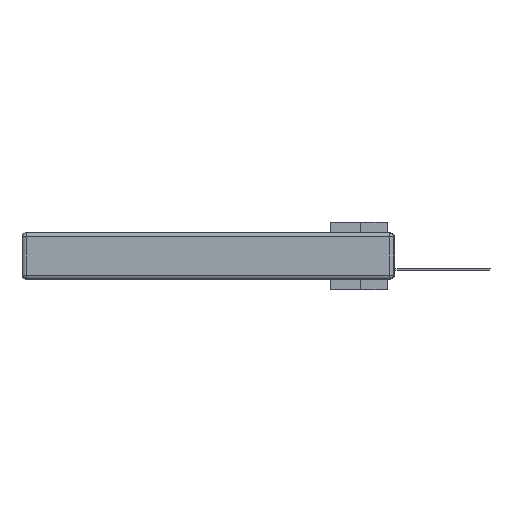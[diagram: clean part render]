
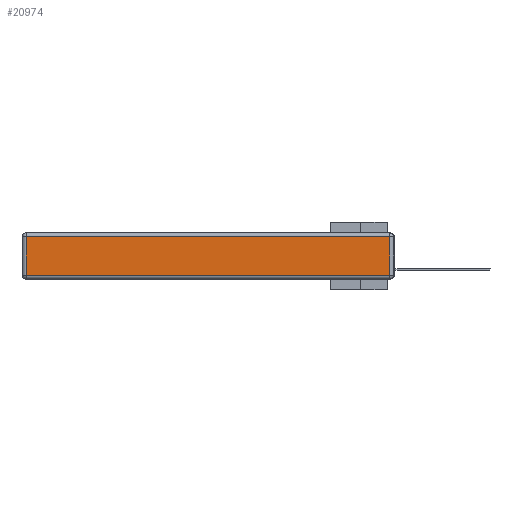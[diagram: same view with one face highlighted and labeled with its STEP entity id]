
A CAD part, left-side view. The second image highlights one B-rep face of the part: STEP entity #20974.
In plain terms, the highlighted planar face has unit normal (-1, 0, 0).
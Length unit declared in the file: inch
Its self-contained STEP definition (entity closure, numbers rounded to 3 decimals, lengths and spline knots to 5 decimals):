
#761 = VECTOR ( 'NONE', #27339, 39.37008 ) ;
#1589 = VECTOR ( 'NONE', #25922, 39.37008 ) ;
#2242 = PLANE ( 'NONE',  #30374 ) ;
#3369 = CARTESIAN_POINT ( 'NONE',  ( 0., 2.72, -0.313 ) ) ;
#3684 = EDGE_CURVE ( 'NONE', #26740, #18772, #24900, .T. ) ;
#3913 = DIRECTION ( 'NONE',  ( 0., -1., 0. ) ) ;
#5776 = EDGE_LOOP ( 'NONE', ( #15739, #10584, #27710, #9105 ) ) ;
#6708 = DIRECTION ( 'NONE',  ( 0., 1., 0. ) ) ;
#7446 = FACE_OUTER_BOUND ( 'NONE', #5776, .T. ) ;
#7836 = VECTOR ( 'NONE', #3913, 39.37008 ) ;
#9105 = ORIENTED_EDGE ( 'NONE', *, *, #3684, .T. ) ;
#9355 = VECTOR ( 'NONE', #6708, 39.37008 ) ;
#10584 = ORIENTED_EDGE ( 'NONE', *, *, #13278, .T. ) ;
#12025 = LINE ( 'NONE', #31526, #7836 ) ;
#13278 = EDGE_CURVE ( 'NONE', #18781, #29137, #26244, .T. ) ;
#13727 = CARTESIAN_POINT ( 'NONE',  ( 0., 0.03, -0.03 ) ) ;
#15739 = ORIENTED_EDGE ( 'NONE', *, *, #31503, .T. ) ;
#16780 = LINE ( 'NONE', #27013, #9355 ) ;
#16877 = DIRECTION ( 'NONE',  ( 0., 0., 1. ) ) ;
#17421 = CARTESIAN_POINT ( 'NONE',  ( 0., 2.72, -0.343 ) ) ;
#17637 = EDGE_CURVE ( 'NONE', #29137, #26740, #16780, .T. ) ;
#18762 = CARTESIAN_POINT ( 'NONE',  ( 0., 0.03, -0.343 ) ) ;
#18772 = VERTEX_POINT ( 'NONE', #3369 ) ;
#18781 = VERTEX_POINT ( 'NONE', #30198 ) ;
#20974 = ADVANCED_FACE ( 'NONE', ( #7446 ), #2242, .T. ) ;
#24526 = CARTESIAN_POINT ( 'NONE',  ( 0., 0., -0.343 ) ) ;
#24900 = LINE ( 'NONE', #17421, #761 ) ;
#25922 = DIRECTION ( 'NONE',  ( 0., 0., 1. ) ) ;
#26244 = LINE ( 'NONE', #18762, #1589 ) ;
#26740 = VERTEX_POINT ( 'NONE', #30286 ) ;
#27013 = CARTESIAN_POINT ( 'NONE',  ( 0., 2.75, -0.03 ) ) ;
#27281 = DIRECTION ( 'NONE',  ( -1., 0., 0. ) ) ;
#27339 = DIRECTION ( 'NONE',  ( 0., 0., -1. ) ) ;
#27710 = ORIENTED_EDGE ( 'NONE', *, *, #17637, .T. ) ;
#29137 = VERTEX_POINT ( 'NONE', #13727 ) ;
#30198 = CARTESIAN_POINT ( 'NONE',  ( 0., 0.03, -0.313 ) ) ;
#30286 = CARTESIAN_POINT ( 'NONE',  ( 0., 2.72, -0.03 ) ) ;
#30374 = AXIS2_PLACEMENT_3D ( 'NONE', #24526, #27281, #16877 ) ;
#31503 = EDGE_CURVE ( 'NONE', #18772, #18781, #12025, .T. ) ;
#31526 = CARTESIAN_POINT ( 'NONE',  ( 0., 0., -0.313 ) ) ;
